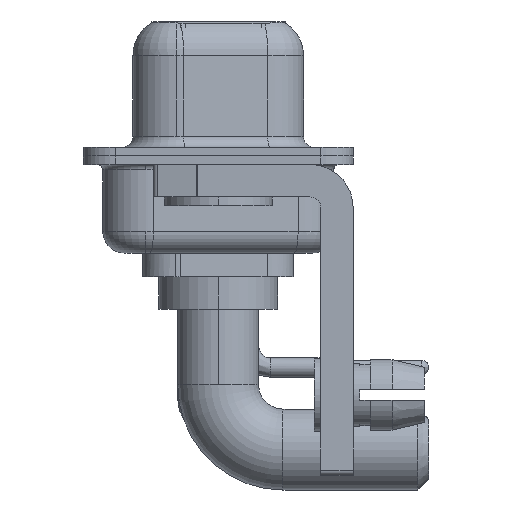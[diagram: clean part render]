
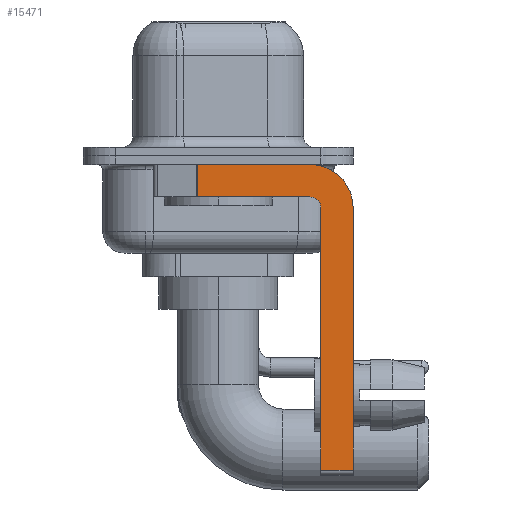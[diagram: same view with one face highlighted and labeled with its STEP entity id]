
A CAD part, left-side view. The second image highlights one B-rep face of the part: STEP entity #15471.
In plain terms, the highlighted planar face has unit normal (-1, 0, 0).
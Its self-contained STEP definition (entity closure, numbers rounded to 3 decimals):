
#115 = VECTOR ( 'NONE', #14415, 1000. ) ;
#429 = CARTESIAN_POINT ( 'NONE',  ( -2.9, 3., -0.4 ) ) ;
#938 = EDGE_CURVE ( 'NONE', #12425, #2558, #26986, .T. ) ;
#1082 = VERTEX_POINT ( 'NONE', #4736 ) ;
#1612 = PLANE ( 'NONE',  #2096 ) ;
#1820 = VECTOR ( 'NONE', #17221, 1000. ) ;
#1876 = LINE ( 'NONE', #6012, #115 ) ;
#1949 = DIRECTION ( 'NONE',  ( 0., 0., 1. ) ) ;
#2096 = AXIS2_PLACEMENT_3D ( 'NONE', #7820, #26385, #24600 ) ;
#2212 = EDGE_CURVE ( 'NONE', #15144, #1082, #1876, .T. ) ;
#2282 = EDGE_CURVE ( 'NONE', #8777, #20907, #10111, .T. ) ;
#2558 = VERTEX_POINT ( 'NONE', #24908 ) ;
#2676 = CARTESIAN_POINT ( 'NONE',  ( -2.9, -4.25, -1.9 ) ) ;
#3069 = ORIENTED_EDGE ( 'NONE', *, *, #9922, .F. ) ;
#3198 = LINE ( 'NONE', #429, #1820 ) ;
#3232 = ORIENTED_EDGE ( 'NONE', *, *, #938, .F. ) ;
#3282 = AXIS2_PLACEMENT_3D ( 'NONE', #27040, #12617, #4334 ) ;
#4011 = CARTESIAN_POINT ( 'NONE',  ( -2.9, -4.25, -2.4 ) ) ;
#4334 = DIRECTION ( 'NONE',  ( 0., 0., -1. ) ) ;
#4736 = CARTESIAN_POINT ( 'NONE',  ( -2.9, -6.25, -14.55 ) ) ;
#5941 = ORIENTED_EDGE ( 'NONE', *, *, #2212, .T. ) ;
#6012 = CARTESIAN_POINT ( 'NONE',  ( -2.9, -4.25, -14.55 ) ) ;
#6627 = DIRECTION ( 'NONE',  ( 0., 0., 1. ) ) ;
#6686 = VECTOR ( 'NONE', #6627, 1000. ) ;
#6938 = CARTESIAN_POINT ( 'NONE',  ( -2.9, -6.25, -2.4 ) ) ;
#7820 = CARTESIAN_POINT ( 'NONE',  ( -2.9, -4.25, -2.4 ) ) ;
#8177 = CARTESIAN_POINT ( 'NONE',  ( -2.9, 0.978, -1.9 ) ) ;
#8777 = VERTEX_POINT ( 'NONE', #18669 ) ;
#9542 = VECTOR ( 'NONE', #15339, 1000. ) ;
#9922 = EDGE_CURVE ( 'NONE', #15144, #8777, #25870, .T. ) ;
#10111 = CIRCLE ( 'NONE', #25896, 0.5 ) ;
#10518 = LINE ( 'NONE', #8177, #14925 ) ;
#10541 = EDGE_LOOP ( 'NONE', ( #17666, #13629, #20038, #19747, #3069, #5941, #12283, #3232 ) ) ;
#12283 = ORIENTED_EDGE ( 'NONE', *, *, #14291, .F. ) ;
#12425 = VERTEX_POINT ( 'NONE', #12907 ) ;
#12617 = DIRECTION ( 'NONE',  ( 1., 0., 0. ) ) ;
#12835 = DIRECTION ( 'NONE',  ( -1., 0., 0. ) ) ;
#12907 = CARTESIAN_POINT ( 'NONE',  ( -2.9, -4.25, -0.4 ) ) ;
#13629 = ORIENTED_EDGE ( 'NONE', *, *, #25200, .T. ) ;
#14070 = CARTESIAN_POINT ( 'NONE',  ( -2.9, -4.25, -1.9 ) ) ;
#14291 = EDGE_CURVE ( 'NONE', #2558, #1082, #19441, .T. ) ;
#14415 = DIRECTION ( 'NONE',  ( 0., -1., 0. ) ) ;
#14776 = CARTESIAN_POINT ( 'NONE',  ( -2.9, 0.978, -0.4 ) ) ;
#14925 = VECTOR ( 'NONE', #18890, 1000. ) ;
#15014 = CARTESIAN_POINT ( 'NONE',  ( -2.9, -4.75, -14.55 ) ) ;
#15144 = VERTEX_POINT ( 'NONE', #15014 ) ;
#15339 = DIRECTION ( 'NONE',  ( 0., 0., -1. ) ) ;
#15471 = ADVANCED_FACE ( 'NONE', ( #26650 ), #1612, .F. ) ;
#17056 = CARTESIAN_POINT ( 'NONE',  ( -2.9, 0.978, -1.9 ) ) ;
#17065 = CARTESIAN_POINT ( 'NONE',  ( -2.9, -4.75, -14.8 ) ) ;
#17221 = DIRECTION ( 'NONE',  ( 0., -1., 0. ) ) ;
#17451 = VERTEX_POINT ( 'NONE', #14776 ) ;
#17666 = ORIENTED_EDGE ( 'NONE', *, *, #20128, .F. ) ;
#18582 = LINE ( 'NONE', #14070, #25301 ) ;
#18669 = CARTESIAN_POINT ( 'NONE',  ( -2.9, -4.75, -2.4 ) ) ;
#18890 = DIRECTION ( 'NONE',  ( 0., 0., -1. ) ) ;
#19441 = LINE ( 'NONE', #6938, #9542 ) ;
#19747 = ORIENTED_EDGE ( 'NONE', *, *, #2282, .F. ) ;
#20038 = ORIENTED_EDGE ( 'NONE', *, *, #24207, .F. ) ;
#20128 = EDGE_CURVE ( 'NONE', #17451, #12425, #3198, .T. ) ;
#20907 = VERTEX_POINT ( 'NONE', #2676 ) ;
#24207 = EDGE_CURVE ( 'NONE', #20907, #25746, #18582, .T. ) ;
#24600 = DIRECTION ( 'NONE',  ( 0., 0., -1. ) ) ;
#24908 = CARTESIAN_POINT ( 'NONE',  ( -2.9, -6.25, -2.4 ) ) ;
#25183 = DIRECTION ( 'NONE',  ( 0., 1., 0. ) ) ;
#25200 = EDGE_CURVE ( 'NONE', #17451, #25746, #10518, .T. ) ;
#25301 = VECTOR ( 'NONE', #25183, 1000. ) ;
#25746 = VERTEX_POINT ( 'NONE', #17056 ) ;
#25870 = LINE ( 'NONE', #17065, #6686 ) ;
#25896 = AXIS2_PLACEMENT_3D ( 'NONE', #4011, #12835, #1949 ) ;
#26385 = DIRECTION ( 'NONE',  ( 1., 0., 0. ) ) ;
#26650 = FACE_OUTER_BOUND ( 'NONE', #10541, .T. ) ;
#26986 = CIRCLE ( 'NONE', #3282, 2. ) ;
#27040 = CARTESIAN_POINT ( 'NONE',  ( -2.9, -4.25, -2.4 ) ) ;
